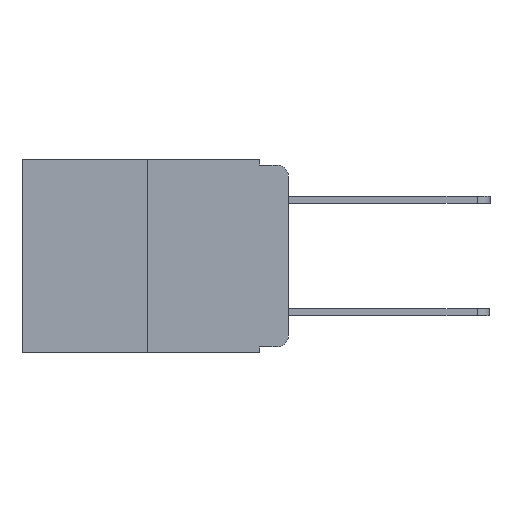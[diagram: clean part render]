
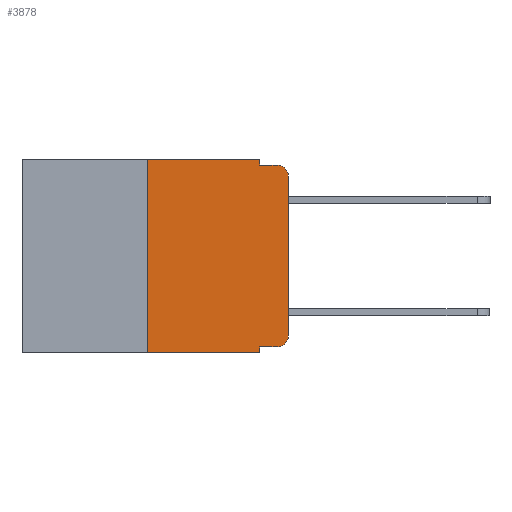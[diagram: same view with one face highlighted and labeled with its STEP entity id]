
A CAD part, left-side view. The second image highlights one B-rep face of the part: STEP entity #3878.
In plain terms, the highlighted planar face has unit normal (-1, 0, 0).
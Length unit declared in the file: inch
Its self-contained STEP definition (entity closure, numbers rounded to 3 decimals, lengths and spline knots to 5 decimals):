
#6 = VERTEX_POINT ( 'NONE', #10497 ) ;
#7 = EDGE_CURVE ( 'NONE', #10892, #4452, #5100, .T. ) ;
#105 = DIRECTION ( 'NONE',  ( 0., -1., 0. ) ) ;
#117 = DIRECTION ( 'NONE',  ( 0., 0., -1. ) ) ;
#152 = ORIENTED_EDGE ( 'NONE', *, *, #7, .T. ) ;
#203 = EDGE_CURVE ( 'NONE', #9677, #10464, #3903, .T. ) ;
#333 = EDGE_LOOP ( 'NONE', ( #11173, #10690, #1251, #5745, #9900, #1265, #152, #7012, #4394, #8893 ) ) ;
#516 = CIRCLE ( 'NONE', #3946, 0.02 ) ;
#540 = CARTESIAN_POINT ( 'NONE',  ( 0., 0., 0. ) ) ;
#627 = CARTESIAN_POINT ( 'NONE',  ( 0., 0.051, -0.01 ) ) ;
#651 = EDGE_CURVE ( 'NONE', #5554, #8231, #11008, .T. ) ;
#947 = CARTESIAN_POINT ( 'NONE',  ( 0., 0.051, 0. ) ) ;
#971 = VERTEX_POINT ( 'NONE', #8782 ) ;
#1251 = ORIENTED_EDGE ( 'NONE', *, *, #203, .F. ) ;
#1265 = ORIENTED_EDGE ( 'NONE', *, *, #3871, .F. ) ;
#1283 = CARTESIAN_POINT ( 'NONE',  ( 0., 0.473, 0. ) ) ;
#1510 = CIRCLE ( 'NONE', #9813, 0.02 ) ;
#1623 = EDGE_CURVE ( 'NONE', #6, #5830, #5491, .T. ) ;
#1749 = EDGE_CURVE ( 'NONE', #8231, #9677, #8406, .T. ) ;
#2536 = VECTOR ( 'NONE', #6123, 39.37008 ) ;
#2705 = DIRECTION ( 'NONE',  ( -1., 0., 0. ) ) ;
#3205 = CARTESIAN_POINT ( 'NONE',  ( 0., 0.02, -0.313 ) ) ;
#3231 = CARTESIAN_POINT ( 'NONE',  ( 0., 0.473, 0. ) ) ;
#3236 = EDGE_CURVE ( 'NONE', #6, #4452, #6708, .T. ) ;
#3262 = DIRECTION ( 'NONE',  ( 1., 0., 0. ) ) ;
#3597 = CARTESIAN_POINT ( 'NONE',  ( 0., 0.25, 0. ) ) ;
#3871 = EDGE_CURVE ( 'NONE', #10892, #5554, #7962, .T. ) ;
#3878 = ADVANCED_FACE ( 'NONE', ( #9888 ), #10180, .F. ) ;
#3903 = LINE ( 'NONE', #627, #8314 ) ;
#3946 = AXIS2_PLACEMENT_3D ( 'NONE', #3205, #9347, #4154 ) ;
#4014 = DIRECTION ( 'NONE',  ( 0., -1., 0. ) ) ;
#4154 = DIRECTION ( 'NONE',  ( 0., 0., -1. ) ) ;
#4248 = VECTOR ( 'NONE', #117, 39.37008 ) ;
#4370 = CARTESIAN_POINT ( 'NONE',  ( 0., 0.051, -0.343 ) ) ;
#4394 = ORIENTED_EDGE ( 'NONE', *, *, #1623, .T. ) ;
#4452 = VERTEX_POINT ( 'NONE', #4370 ) ;
#4505 = CARTESIAN_POINT ( 'NONE',  ( 0., 0.051, -0.333 ) ) ;
#5100 = LINE ( 'NONE', #9349, #2536 ) ;
#5481 = DIRECTION ( 'NONE',  ( 0., -1., 0. ) ) ;
#5491 = LINE ( 'NONE', #4505, #7777 ) ;
#5554 = VERTEX_POINT ( 'NONE', #3597 ) ;
#5745 = ORIENTED_EDGE ( 'NONE', *, *, #1749, .F. ) ;
#5785 = CARTESIAN_POINT ( 'NONE',  ( 0., 0.051, 0. ) ) ;
#5830 = VERTEX_POINT ( 'NONE', #6935 ) ;
#5941 = VECTOR ( 'NONE', #6633, 39.37008 ) ;
#5980 = VERTEX_POINT ( 'NONE', #6380 ) ;
#6009 = EDGE_CURVE ( 'NONE', #971, #10464, #1510, .T. ) ;
#6027 = VECTOR ( 'NONE', #10395, 39.37008 ) ;
#6123 = DIRECTION ( 'NONE',  ( 0., -1., 0. ) ) ;
#6380 = CARTESIAN_POINT ( 'NONE',  ( 0., 0., -0.313 ) ) ;
#6420 = AXIS2_PLACEMENT_3D ( 'NONE', #3231, #3262, #9396 ) ;
#6522 = CARTESIAN_POINT ( 'NONE',  ( 0., 0.02, -0.01 ) ) ;
#6611 = CARTESIAN_POINT ( 'NONE',  ( 0., 0.051, -0.01 ) ) ;
#6633 = DIRECTION ( 'NONE',  ( 0., 0., -1. ) ) ;
#6708 = LINE ( 'NONE', #9974, #4248 ) ;
#6935 = CARTESIAN_POINT ( 'NONE',  ( 0., 0.02, -0.333 ) ) ;
#7012 = ORIENTED_EDGE ( 'NONE', *, *, #3236, .F. ) ;
#7718 = VECTOR ( 'NONE', #7754, 39.37008 ) ;
#7754 = DIRECTION ( 'NONE',  ( 0., 0., 1. ) ) ;
#7777 = VECTOR ( 'NONE', #5481, 39.37008 ) ;
#7962 = LINE ( 'NONE', #11017, #7718 ) ;
#8099 = CARTESIAN_POINT ( 'NONE',  ( 0., 0.02, -0.03 ) ) ;
#8231 = VERTEX_POINT ( 'NONE', #5785 ) ;
#8239 = LINE ( 'NONE', #540, #6027 ) ;
#8314 = VECTOR ( 'NONE', #4014, 39.37008 ) ;
#8406 = LINE ( 'NONE', #947, #5941 ) ;
#8440 = EDGE_CURVE ( 'NONE', #5830, #5980, #516, .T. ) ;
#8782 = CARTESIAN_POINT ( 'NONE',  ( 0., 0., -0.03 ) ) ;
#8818 = VECTOR ( 'NONE', #105, 39.37008 ) ;
#8893 = ORIENTED_EDGE ( 'NONE', *, *, #8440, .T. ) ;
#8935 = DIRECTION ( 'NONE',  ( 0., 0., -1. ) ) ;
#9347 = DIRECTION ( 'NONE',  ( -1., 0., 0. ) ) ;
#9349 = CARTESIAN_POINT ( 'NONE',  ( 0., 0.473, -0.343 ) ) ;
#9378 = CARTESIAN_POINT ( 'NONE',  ( 0., 0.25, -0.343 ) ) ;
#9396 = DIRECTION ( 'NONE',  ( 0., 0., -1. ) ) ;
#9677 = VERTEX_POINT ( 'NONE', #6611 ) ;
#9813 = AXIS2_PLACEMENT_3D ( 'NONE', #8099, #2705, #8935 ) ;
#9888 = FACE_OUTER_BOUND ( 'NONE', #333, .T. ) ;
#9900 = ORIENTED_EDGE ( 'NONE', *, *, #651, .F. ) ;
#9974 = CARTESIAN_POINT ( 'NONE',  ( 0., 0.051, 0. ) ) ;
#10180 = PLANE ( 'NONE',  #6420 ) ;
#10219 = EDGE_CURVE ( 'NONE', #5980, #971, #8239, .T. ) ;
#10395 = DIRECTION ( 'NONE',  ( 0., 0., 1. ) ) ;
#10464 = VERTEX_POINT ( 'NONE', #6522 ) ;
#10497 = CARTESIAN_POINT ( 'NONE',  ( 0., 0.051, -0.333 ) ) ;
#10690 = ORIENTED_EDGE ( 'NONE', *, *, #6009, .T. ) ;
#10892 = VERTEX_POINT ( 'NONE', #9378 ) ;
#11008 = LINE ( 'NONE', #1283, #8818 ) ;
#11017 = CARTESIAN_POINT ( 'NONE',  ( 0., 0.25, 0. ) ) ;
#11173 = ORIENTED_EDGE ( 'NONE', *, *, #10219, .T. ) ;
